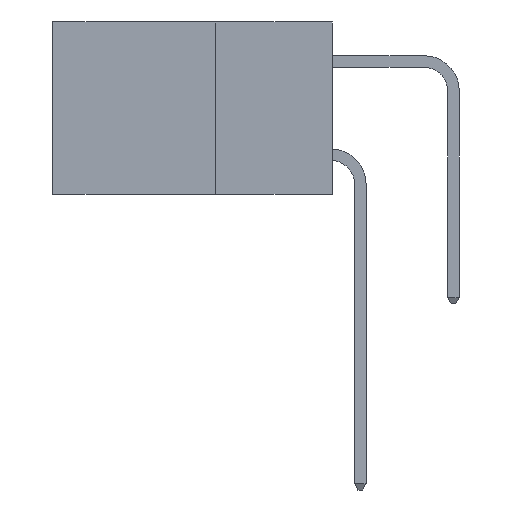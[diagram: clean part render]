
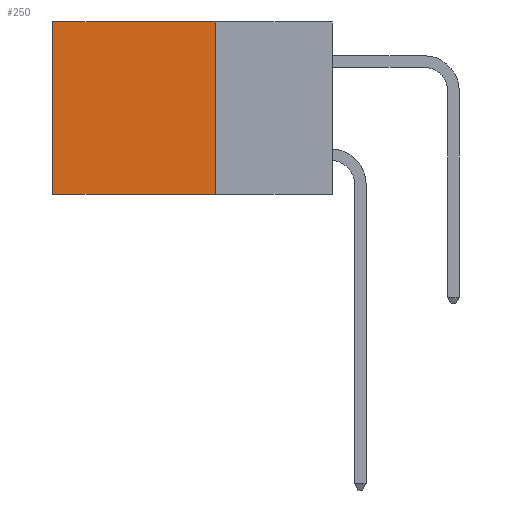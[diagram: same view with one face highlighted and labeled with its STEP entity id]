
A CAD part, left-side view. The second image highlights one B-rep face of the part: STEP entity #250.
In plain terms, the highlighted planar face has unit normal (-1, 0, 0).
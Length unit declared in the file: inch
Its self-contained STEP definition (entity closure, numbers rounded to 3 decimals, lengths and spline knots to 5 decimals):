
#250 = ADVANCED_FACE ( 'NONE', ( #13622 ), #4733, .F. ) ;
#1653 = VECTOR ( 'NONE', #12007, 39.37008 ) ;
#1995 = ORIENTED_EDGE ( 'NONE', *, *, #11546, .T. ) ;
#4046 = DIRECTION ( 'NONE',  ( 0., 0., -1. ) ) ;
#4171 = ORIENTED_EDGE ( 'NONE', *, *, #7948, .T. ) ;
#4733 = PLANE ( 'NONE',  #18213 ) ;
#5104 = ORIENTED_EDGE ( 'NONE', *, *, #12311, .F. ) ;
#6415 = CARTESIAN_POINT ( 'NONE',  ( 0.2615, 0.25, -0.37 ) ) ;
#6892 = VERTEX_POINT ( 'NONE', #24564 ) ;
#7925 = CARTESIAN_POINT ( 'NONE',  ( 0.2615, 0.25, 0. ) ) ;
#7948 = EDGE_CURVE ( 'NONE', #14743, #21118, #23663, .T. ) ;
#8612 = CARTESIAN_POINT ( 'NONE',  ( 0.2615, 0.25, -0.37 ) ) ;
#9229 = DIRECTION ( 'NONE',  ( 1., 0., 0. ) ) ;
#9887 = CARTESIAN_POINT ( 'NONE',  ( 0.2615, 0.25, 0. ) ) ;
#11546 = EDGE_CURVE ( 'NONE', #16464, #14743, #18613, .T. ) ;
#11713 = VECTOR ( 'NONE', #26980, 39.37008 ) ;
#11925 = VECTOR ( 'NONE', #23526, 39.37008 ) ;
#12007 = DIRECTION ( 'NONE',  ( 0., 1., 0. ) ) ;
#12311 = EDGE_CURVE ( 'NONE', #16464, #6892, #22804, .T. ) ;
#12764 = EDGE_LOOP ( 'NONE', ( #4171, #14930, #5104, #1995 ) ) ;
#12876 = DIRECTION ( 'NONE',  ( 0., 1., 0. ) ) ;
#12973 = VECTOR ( 'NONE', #12876, 39.37008 ) ;
#13103 = EDGE_CURVE ( 'NONE', #6892, #21118, #18567, .T. ) ;
#13622 = FACE_OUTER_BOUND ( 'NONE', #12764, .T. ) ;
#14743 = VERTEX_POINT ( 'NONE', #26330 ) ;
#14930 = ORIENTED_EDGE ( 'NONE', *, *, #13103, .F. ) ;
#16464 = VERTEX_POINT ( 'NONE', #7925 ) ;
#18213 = AXIS2_PLACEMENT_3D ( 'NONE', #6415, #9229, #4046 ) ;
#18567 = LINE ( 'NONE', #8612, #12973 ) ;
#18613 = LINE ( 'NONE', #9887, #1653 ) ;
#18777 = CARTESIAN_POINT ( 'NONE',  ( 0.2615, 0.25, -0.37 ) ) ;
#21118 = VERTEX_POINT ( 'NONE', #26562 ) ;
#21442 = CARTESIAN_POINT ( 'NONE',  ( 0.2615, 0.6, -0.37 ) ) ;
#22804 = LINE ( 'NONE', #18777, #11713 ) ;
#23526 = DIRECTION ( 'NONE',  ( 0., 0., -1. ) ) ;
#23663 = LINE ( 'NONE', #21442, #11925 ) ;
#24564 = CARTESIAN_POINT ( 'NONE',  ( 0.2615, 0.25, -0.37 ) ) ;
#26330 = CARTESIAN_POINT ( 'NONE',  ( 0.2615, 0.6, 0. ) ) ;
#26562 = CARTESIAN_POINT ( 'NONE',  ( 0.2615, 0.6, -0.37 ) ) ;
#26980 = DIRECTION ( 'NONE',  ( 0., 0., -1. ) ) ;
